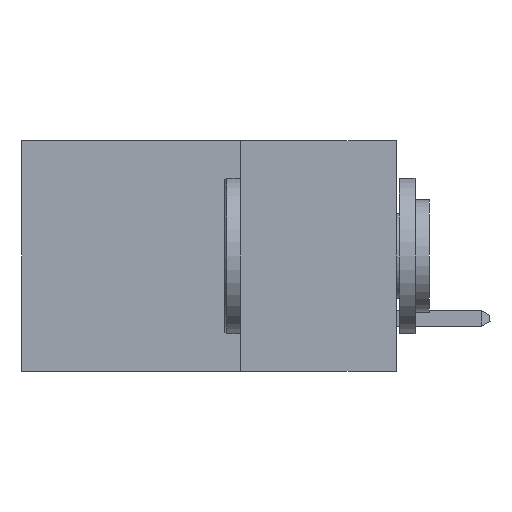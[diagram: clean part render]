
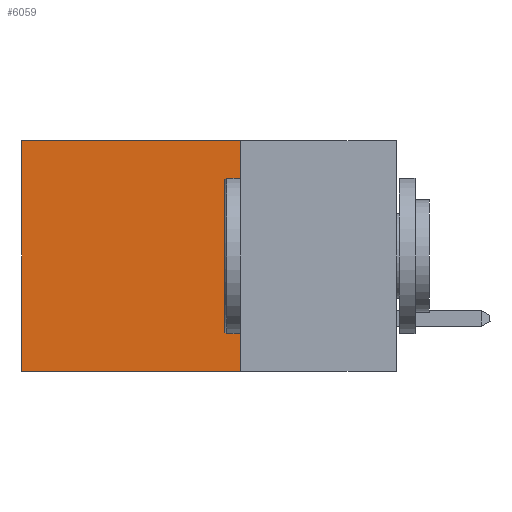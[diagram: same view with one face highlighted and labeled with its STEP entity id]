
A CAD part, left-side view. The second image highlights one B-rep face of the part: STEP entity #6059.
In plain terms, the highlighted planar face has unit normal (-1, 0, 0).
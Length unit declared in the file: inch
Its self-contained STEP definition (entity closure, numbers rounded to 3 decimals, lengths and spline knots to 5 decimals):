
#608 = EDGE_CURVE ( 'NONE', #10898, #9319, #12259, .T. ) ;
#909 = CARTESIAN_POINT ( 'NONE',  ( 0.298, 0.25, 0. ) ) ;
#1303 = VECTOR ( 'NONE', #11556, 39.37008 ) ;
#1399 = VERTEX_POINT ( 'NONE', #1893 ) ;
#1893 = CARTESIAN_POINT ( 'NONE',  ( 0.298, 0.25, -0.37 ) ) ;
#2017 = FACE_OUTER_BOUND ( 'NONE', #4073, .T. ) ;
#2060 = ORIENTED_EDGE ( 'NONE', *, *, #11147, .F. ) ;
#2295 = VERTEX_POINT ( 'NONE', #909 ) ;
#2329 = CARTESIAN_POINT ( 'NONE',  ( 0.298, 0.25, 0. ) ) ;
#2458 = CARTESIAN_POINT ( 'NONE',  ( 0.298, 0.25, 0. ) ) ;
#2597 = AXIS2_PLACEMENT_3D ( 'NONE', #2458, #3425, #9966 ) ;
#3293 = DIRECTION ( 'NONE',  ( 0., 0., -1. ) ) ;
#3425 = DIRECTION ( 'NONE',  ( 1., 0., 0. ) ) ;
#3458 = EDGE_CURVE ( 'NONE', #1399, #9319, #9474, .T. ) ;
#3938 = CARTESIAN_POINT ( 'NONE',  ( 0.298, 0.6, 0. ) ) ;
#4073 = EDGE_LOOP ( 'NONE', ( #10844, #4330, #2060, #9582 ) ) ;
#4330 = ORIENTED_EDGE ( 'NONE', *, *, #3458, .F. ) ;
#4765 = LINE ( 'NONE', #2329, #9432 ) ;
#5079 = CARTESIAN_POINT ( 'NONE',  ( 0.298, 0.25, 0. ) ) ;
#6059 = ADVANCED_FACE ( 'NONE', ( #2017 ), #9012, .F. ) ;
#6151 = CARTESIAN_POINT ( 'NONE',  ( 0.298, 0.6, -0.37 ) ) ;
#7557 = CARTESIAN_POINT ( 'NONE',  ( 0.298, 0.25, -0.37 ) ) ;
#8339 = CARTESIAN_POINT ( 'NONE',  ( 0.298, 0.6, 0. ) ) ;
#8567 = LINE ( 'NONE', #5079, #1303 ) ;
#8809 = DIRECTION ( 'NONE',  ( 0., 0., -1. ) ) ;
#9012 = PLANE ( 'NONE',  #2597 ) ;
#9319 = VERTEX_POINT ( 'NONE', #6151 ) ;
#9422 = DIRECTION ( 'NONE',  ( 0., 1., 0. ) ) ;
#9432 = VECTOR ( 'NONE', #3293, 39.37008 ) ;
#9474 = LINE ( 'NONE', #7557, #11908 ) ;
#9582 = ORIENTED_EDGE ( 'NONE', *, *, #9871, .T. ) ;
#9871 = EDGE_CURVE ( 'NONE', #2295, #10898, #8567, .T. ) ;
#9966 = DIRECTION ( 'NONE',  ( 0., 0., -1. ) ) ;
#10844 = ORIENTED_EDGE ( 'NONE', *, *, #608, .T. ) ;
#10898 = VERTEX_POINT ( 'NONE', #3938 ) ;
#11147 = EDGE_CURVE ( 'NONE', #2295, #1399, #4765, .T. ) ;
#11556 = DIRECTION ( 'NONE',  ( 0., 1., 0. ) ) ;
#11908 = VECTOR ( 'NONE', #9422, 39.37008 ) ;
#11966 = VECTOR ( 'NONE', #8809, 39.37008 ) ;
#12259 = LINE ( 'NONE', #8339, #11966 ) ;
